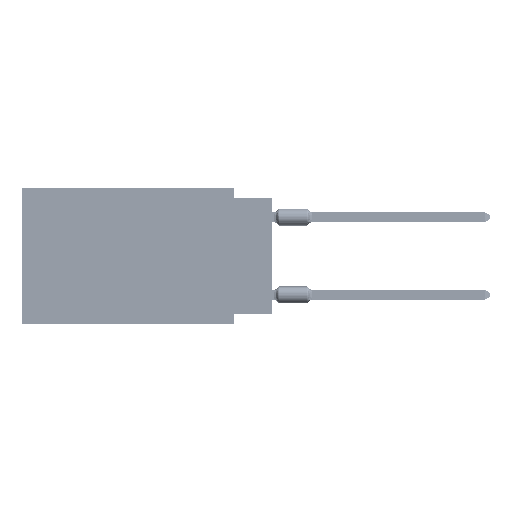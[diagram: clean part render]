
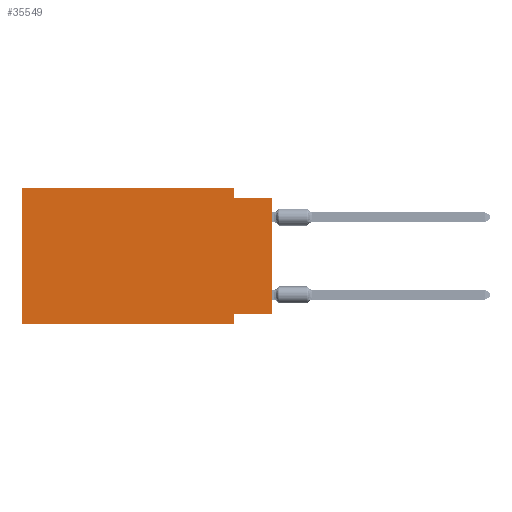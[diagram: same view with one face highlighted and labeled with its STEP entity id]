
A CAD part, left-side view. The second image highlights one B-rep face of the part: STEP entity #35549.
In plain terms, the highlighted planar face has unit normal (-1, 0, 0).
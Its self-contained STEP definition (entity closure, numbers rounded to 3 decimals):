
#175 = EDGE_CURVE ( 'NONE', #11061, #7510, #8614, .T. ) ;
#2790 = DIRECTION ( 'NONE',  ( 0., 0., 1. ) ) ;
#3789 = PLANE ( 'NONE',  #60518 ) ;
#6152 = CARTESIAN_POINT ( 'NONE',  ( 0., 2.54, 0. ) ) ;
#7096 = VERTEX_POINT ( 'NONE', #15585 ) ;
#7510 = VERTEX_POINT ( 'NONE', #74752 ) ;
#8614 = LINE ( 'NONE', #42619, #68152 ) ;
#9403 = VERTEX_POINT ( 'NONE', #6152 ) ;
#11061 = VERTEX_POINT ( 'NONE', #81652 ) ;
#15238 = ORIENTED_EDGE ( 'NONE', *, *, #16112, .F. ) ;
#15585 = CARTESIAN_POINT ( 'NONE',  ( 0., 0., -0.635 ) ) ;
#16112 = EDGE_CURVE ( 'NONE', #7510, #42697, #43395, .T. ) ;
#16873 = CARTESIAN_POINT ( 'NONE',  ( 0., 0., -0.635 ) ) ;
#17647 = CARTESIAN_POINT ( 'NONE',  ( 0., 2.54, -8.89 ) ) ;
#21765 = CARTESIAN_POINT ( 'NONE',  ( 0., 16.383, 0. ) ) ;
#22008 = ORIENTED_EDGE ( 'NONE', *, *, #41475, .F. ) ;
#24709 = DIRECTION ( 'NONE',  ( 1., 0., 0. ) ) ;
#25851 = LINE ( 'NONE', #44648, #59124 ) ;
#29175 = CARTESIAN_POINT ( 'NONE',  ( 0., 16.383, -8.89 ) ) ;
#29819 = CARTESIAN_POINT ( 'NONE',  ( 0., 0., 0. ) ) ;
#30831 = DIRECTION ( 'NONE',  ( 0., 0., -1. ) ) ;
#31685 = FACE_OUTER_BOUND ( 'NONE', #79539, .T. ) ;
#35549 = ADVANCED_FACE ( 'NONE', ( #31685 ), #3789, .F. ) ;
#35552 = CARTESIAN_POINT ( 'NONE',  ( 0., 16.383, -8.89 ) ) ;
#35931 = LINE ( 'NONE', #29819, #70469 ) ;
#37058 = VERTEX_POINT ( 'NONE', #35552 ) ;
#41315 = VERTEX_POINT ( 'NONE', #45369 ) ;
#41475 = EDGE_CURVE ( 'NONE', #41315, #9403, #81059, .T. ) ;
#41844 = DIRECTION ( 'NONE',  ( 0., -1., 0. ) ) ;
#42235 = VECTOR ( 'NONE', #82774, 1000. ) ;
#42619 = CARTESIAN_POINT ( 'NONE',  ( 0., 0., -8.255 ) ) ;
#42697 = VERTEX_POINT ( 'NONE', #66485 ) ;
#42709 = LINE ( 'NONE', #29175, #42235 ) ;
#43395 = LINE ( 'NONE', #17647, #45867 ) ;
#44648 = CARTESIAN_POINT ( 'NONE',  ( 0., 16.383, 0. ) ) ;
#45369 = CARTESIAN_POINT ( 'NONE',  ( 0., 16.383, 0. ) ) ;
#45867 = VECTOR ( 'NONE', #57761, 1000. ) ;
#50880 = CARTESIAN_POINT ( 'NONE',  ( 0., 16.383, 0. ) ) ;
#52455 = DIRECTION ( 'NONE',  ( 0., 0., 1. ) ) ;
#52457 = ORIENTED_EDGE ( 'NONE', *, *, #175, .F. ) ;
#55129 = ORIENTED_EDGE ( 'NONE', *, *, #83042, .F. ) ;
#57761 = DIRECTION ( 'NONE',  ( 0., 0., -1. ) ) ;
#58423 = VERTEX_POINT ( 'NONE', #61332 ) ;
#59124 = VECTOR ( 'NONE', #52455, 1000. ) ;
#60182 = VECTOR ( 'NONE', #41844, 1000. ) ;
#60518 = AXIS2_PLACEMENT_3D ( 'NONE', #50880, #24709, #30831 ) ;
#61332 = CARTESIAN_POINT ( 'NONE',  ( 0., 2.54, -0.635 ) ) ;
#62080 = CARTESIAN_POINT ( 'NONE',  ( 0., 2.54, 0. ) ) ;
#64380 = DIRECTION ( 'NONE',  ( 0., -1., 0. ) ) ;
#65903 = EDGE_CURVE ( 'NONE', #37058, #42697, #42709, .T. ) ;
#66485 = CARTESIAN_POINT ( 'NONE',  ( 0., 2.54, -8.89 ) ) ;
#68152 = VECTOR ( 'NONE', #69184, 1000. ) ;
#69184 = DIRECTION ( 'NONE',  ( 0., 1., 0. ) ) ;
#69255 = EDGE_CURVE ( 'NONE', #37058, #41315, #25851, .T. ) ;
#69903 = DIRECTION ( 'NONE',  ( 0., 0., -1. ) ) ;
#70469 = VECTOR ( 'NONE', #2790, 1000. ) ;
#71392 = ORIENTED_EDGE ( 'NONE', *, *, #84717, .T. ) ;
#73022 = VECTOR ( 'NONE', #69903, 1000. ) ;
#74719 = LINE ( 'NONE', #62080, #73022 ) ;
#74752 = CARTESIAN_POINT ( 'NONE',  ( 0., 2.54, -8.255 ) ) ;
#77260 = ORIENTED_EDGE ( 'NONE', *, *, #79867, .F. ) ;
#77881 = LINE ( 'NONE', #16873, #80992 ) ;
#78083 = ORIENTED_EDGE ( 'NONE', *, *, #69255, .F. ) ;
#79539 = EDGE_LOOP ( 'NONE', ( #71392, #77260, #55129, #22008, #78083, #81099, #15238, #52457 ) ) ;
#79867 = EDGE_CURVE ( 'NONE', #58423, #7096, #77881, .T. ) ;
#80992 = VECTOR ( 'NONE', #64380, 1000. ) ;
#81059 = LINE ( 'NONE', #21765, #60182 ) ;
#81099 = ORIENTED_EDGE ( 'NONE', *, *, #65903, .T. ) ;
#81652 = CARTESIAN_POINT ( 'NONE',  ( 0., 0., -8.255 ) ) ;
#82774 = DIRECTION ( 'NONE',  ( 0., -1., 0. ) ) ;
#83042 = EDGE_CURVE ( 'NONE', #9403, #58423, #74719, .T. ) ;
#84717 = EDGE_CURVE ( 'NONE', #11061, #7096, #35931, .T. ) ;
